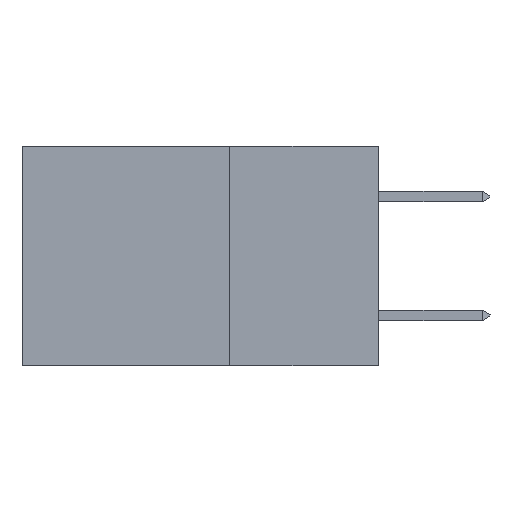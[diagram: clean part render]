
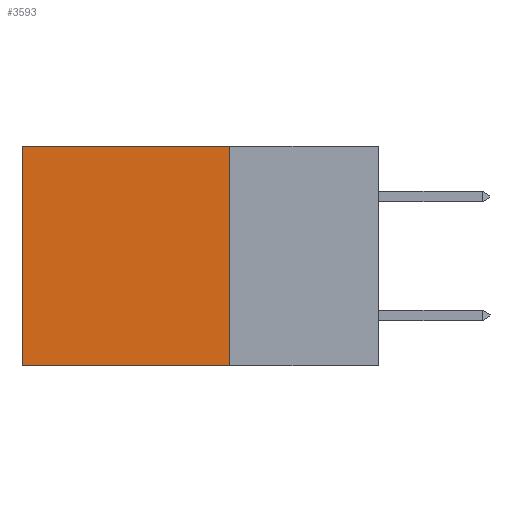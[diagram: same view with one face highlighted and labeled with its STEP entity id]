
A CAD part, left-side view. The second image highlights one B-rep face of the part: STEP entity #3593.
In plain terms, the highlighted planar face has unit normal (-1, 0, 0).
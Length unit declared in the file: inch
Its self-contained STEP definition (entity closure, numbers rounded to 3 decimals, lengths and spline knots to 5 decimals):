
#252 = CARTESIAN_POINT ( 'NONE',  ( 0.298, 0.6, 0. ) ) ;
#460 = PLANE ( 'NONE',  #4971 ) ;
#1103 = EDGE_CURVE ( 'NONE', #11956, #8859, #4751, .T. ) ;
#1164 = CARTESIAN_POINT ( 'NONE',  ( 0.298, 0.25, 0. ) ) ;
#1476 = EDGE_LOOP ( 'NONE', ( #10213, #5640, #3462, #1680 ) ) ;
#1592 = CARTESIAN_POINT ( 'NONE',  ( 0.298, 0.25, -0.37 ) ) ;
#1680 = ORIENTED_EDGE ( 'NONE', *, *, #2640, .T. ) ;
#1699 = CARTESIAN_POINT ( 'NONE',  ( 0.298, 0.25, 0. ) ) ;
#2625 = EDGE_CURVE ( 'NONE', #9708, #8859, #4570, .T. ) ;
#2640 = EDGE_CURVE ( 'NONE', #11840, #9708, #2994, .T. ) ;
#2994 = LINE ( 'NONE', #1699, #11834 ) ;
#3462 = ORIENTED_EDGE ( 'NONE', *, *, #10160, .F. ) ;
#3593 = ADVANCED_FACE ( 'NONE', ( #11259 ), #460, .F. ) ;
#3994 = VECTOR ( 'NONE', #7194, 39.37008 ) ;
#4570 = LINE ( 'NONE', #6300, #3994 ) ;
#4751 = LINE ( 'NONE', #1592, #9129 ) ;
#4971 = AXIS2_PLACEMENT_3D ( 'NONE', #5925, #8844, #8679 ) ;
#5640 = ORIENTED_EDGE ( 'NONE', *, *, #1103, .F. ) ;
#5925 = CARTESIAN_POINT ( 'NONE',  ( 0.298, 0.25, 0. ) ) ;
#6181 = DIRECTION ( 'NONE',  ( 0., 1., 0. ) ) ;
#6300 = CARTESIAN_POINT ( 'NONE',  ( 0.298, 0.6, 0. ) ) ;
#6652 = CARTESIAN_POINT ( 'NONE',  ( 0.298, 0.6, -0.37 ) ) ;
#6669 = LINE ( 'NONE', #1164, #11201 ) ;
#7194 = DIRECTION ( 'NONE',  ( 0., 0., -1. ) ) ;
#7807 = DIRECTION ( 'NONE',  ( 0., 0., -1. ) ) ;
#8007 = DIRECTION ( 'NONE',  ( 0., 1., 0. ) ) ;
#8161 = CARTESIAN_POINT ( 'NONE',  ( 0.298, 0.25, 0. ) ) ;
#8679 = DIRECTION ( 'NONE',  ( 0., 0., -1. ) ) ;
#8844 = DIRECTION ( 'NONE',  ( 1., 0., 0. ) ) ;
#8859 = VERTEX_POINT ( 'NONE', #6652 ) ;
#9129 = VECTOR ( 'NONE', #8007, 39.37008 ) ;
#9708 = VERTEX_POINT ( 'NONE', #252 ) ;
#10160 = EDGE_CURVE ( 'NONE', #11840, #11956, #6669, .T. ) ;
#10213 = ORIENTED_EDGE ( 'NONE', *, *, #2625, .T. ) ;
#11082 = CARTESIAN_POINT ( 'NONE',  ( 0.298, 0.25, -0.37 ) ) ;
#11201 = VECTOR ( 'NONE', #7807, 39.37008 ) ;
#11259 = FACE_OUTER_BOUND ( 'NONE', #1476, .T. ) ;
#11834 = VECTOR ( 'NONE', #6181, 39.37008 ) ;
#11840 = VERTEX_POINT ( 'NONE', #8161 ) ;
#11956 = VERTEX_POINT ( 'NONE', #11082 ) ;
